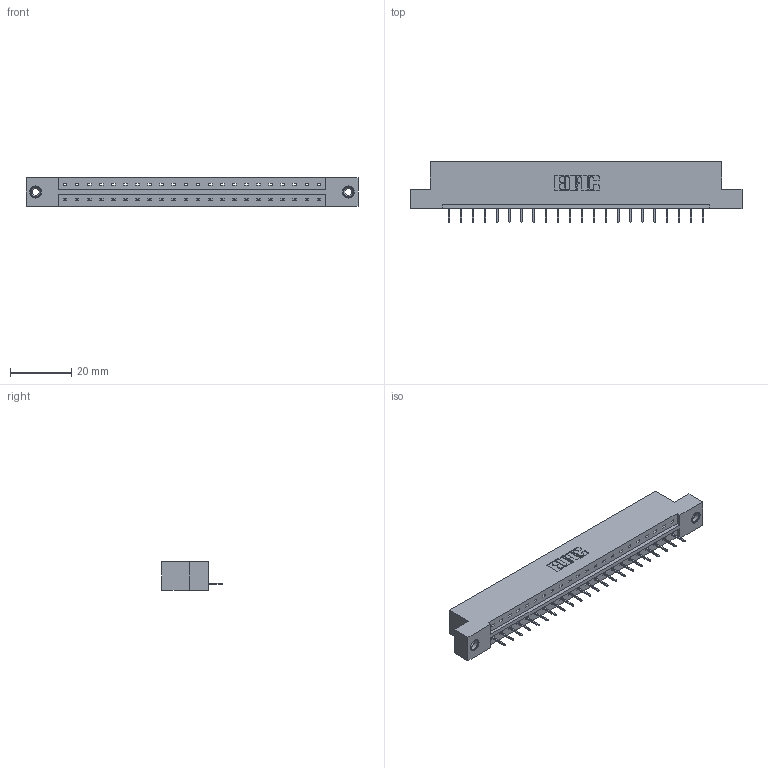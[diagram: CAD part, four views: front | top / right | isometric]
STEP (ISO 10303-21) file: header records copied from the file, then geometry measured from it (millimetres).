
FILE_DESCRIPTION (( 'STEP AP203' ), '1' );
FILE_NAME ('333-022-524-108.STEP', '2018-08-02T01:59:39', ( '' ), ( '' ), 'SwSTEP 2.0', 'SolidWorks 2016', '' );
FILE_SCHEMA (( 'CONFIG_CONTROL_DESIGN' ));
Length unit declared in the file: inch
Products named in the file (4): 333 Part_Flush - .156 Dia - TI; 345-292-001_345-293-124; 345-250-001_345-250-003-102; 333-022-524-108
Assembly tree (25 placements, depth 2):
  333-022-524-108
    333 Part_Flush - .156 Dia - TI
    345-292-001_345-293-124  x22
    345-250-001_345-250-003-102  x2
Bounding box: 108.71 x 19.69 x 9.4 mm (x, y, z)
Volume: 10674.1 mm3; surface area: 11145.4 mm2
Topology: 25 solids, 25 shells, 1538 faces, 4407 edges, 2842 vertices
Faces by surface type: plane 1158, cylinder 364, cone 12, torus 4
Entity records: 17296 total; most frequent: CARTESIAN_POINT 2967, ORIENTED_EDGE 2918, DIRECTION 2577, EDGE_CURVE 1459, VECTOR 1315, LINE 1315, VERTEX_POINT 964, AXIS2_PLACEMENT_3D 631
